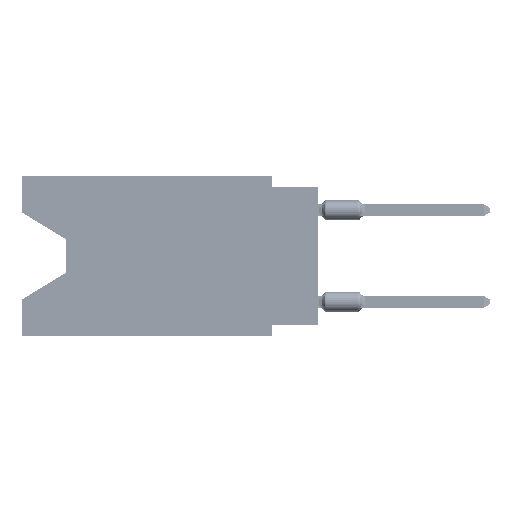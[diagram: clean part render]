
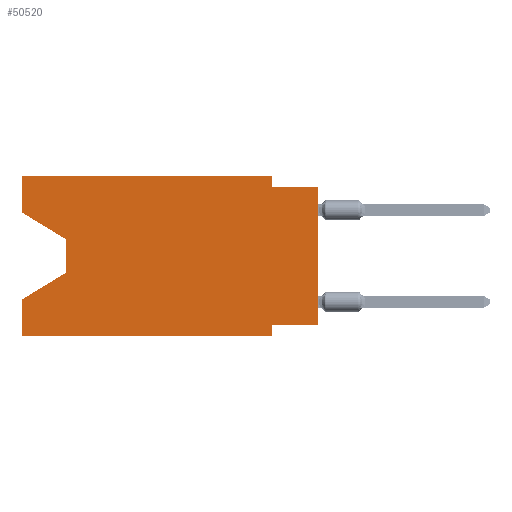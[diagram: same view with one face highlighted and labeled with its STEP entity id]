
A CAD part, left-side view. The second image highlights one B-rep face of the part: STEP entity #50520.
In plain terms, the highlighted planar face has unit normal (-1, 0, 0).
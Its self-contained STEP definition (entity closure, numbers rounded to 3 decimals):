
#161 = LINE ( 'NONE', #12127, #53376 ) ;
#1389 = VECTOR ( 'NONE', #43914, 1000. ) ;
#1641 = LINE ( 'NONE', #44809, #1389 ) ;
#2248 = EDGE_LOOP ( 'NONE', ( #59812, #13426, #54206, #58978, #23460, #26649, #7965, #26960, #28884, #45983, #70749, #5199 ) ) ;
#3345 = VECTOR ( 'NONE', #57295, 1000. ) ;
#5199 = ORIENTED_EDGE ( 'NONE', *, *, #15445, .F. ) ;
#7042 = DIRECTION ( 'NONE',  ( 0., 0., 1. ) ) ;
#7626 = DIRECTION ( 'NONE',  ( 0., 0.855, -0.519 ) ) ;
#7965 = ORIENTED_EDGE ( 'NONE', *, *, #70146, .F. ) ;
#9611 = VECTOR ( 'NONE', #7626, 1000. ) ;
#10541 = CARTESIAN_POINT ( 'NONE',  ( 0., 0., -0.635 ) ) ;
#10916 = DIRECTION ( 'NONE',  ( 0., 1., 0. ) ) ;
#10945 = DIRECTION ( 'NONE',  ( 0., -1., 0. ) ) ;
#11684 = VECTOR ( 'NONE', #10916, 1000. ) ;
#12127 = CARTESIAN_POINT ( 'NONE',  ( 0., 16.383, 0. ) ) ;
#12243 = VECTOR ( 'NONE', #10945, 1000. ) ;
#12475 = EDGE_CURVE ( 'NONE', #48709, #77872, #28798, .T. ) ;
#13426 = ORIENTED_EDGE ( 'NONE', *, *, #64429, .T. ) ;
#15445 = EDGE_CURVE ( 'NONE', #65819, #48709, #1641, .T. ) ;
#17161 = DIRECTION ( 'NONE',  ( 0., 0., -1. ) ) ;
#17624 = LINE ( 'NONE', #74138, #35516 ) ;
#19048 = LINE ( 'NONE', #75562, #59795 ) ;
#19210 = LINE ( 'NONE', #73902, #12243 ) ;
#19377 = CARTESIAN_POINT ( 'NONE',  ( 0., 2.54, -8.255 ) ) ;
#19609 = AXIS2_PLACEMENT_3D ( 'NONE', #20491, #35161, #41598 ) ;
#20093 = VECTOR ( 'NONE', #58358, 1000. ) ;
#20491 = CARTESIAN_POINT ( 'NONE',  ( 0., 16.383, 0. ) ) ;
#23460 = ORIENTED_EDGE ( 'NONE', *, *, #77957, .T. ) ;
#25932 = DIRECTION ( 'NONE',  ( 0., -0.855, -0.519 ) ) ;
#26649 = ORIENTED_EDGE ( 'NONE', *, *, #27356, .F. ) ;
#26960 = ORIENTED_EDGE ( 'NONE', *, *, #90694, .T. ) ;
#27356 = EDGE_CURVE ( 'NONE', #56264, #39975, #40721, .T. ) ;
#27609 = CARTESIAN_POINT ( 'NONE',  ( 0., 13.97, -3.505 ) ) ;
#28172 = CARTESIAN_POINT ( 'NONE',  ( 0., 16.383, -2.038 ) ) ;
#28798 = LINE ( 'NONE', #78430, #3345 ) ;
#28884 = ORIENTED_EDGE ( 'NONE', *, *, #64665, .F. ) ;
#30377 = VERTEX_POINT ( 'NONE', #51569 ) ;
#30771 = LINE ( 'NONE', #10541, #20093 ) ;
#31588 = CARTESIAN_POINT ( 'NONE',  ( 0., 16.383, -6.852 ) ) ;
#32415 = CARTESIAN_POINT ( 'NONE',  ( 0., 0., -0.635 ) ) ;
#35161 = DIRECTION ( 'NONE',  ( 1., 0., 0. ) ) ;
#35516 = VECTOR ( 'NONE', #17161, 1000. ) ;
#36182 = VERTEX_POINT ( 'NONE', #31588 ) ;
#36386 = LINE ( 'NONE', #86483, #37163 ) ;
#37163 = VECTOR ( 'NONE', #50186, 1000. ) ;
#39975 = VERTEX_POINT ( 'NONE', #74692 ) ;
#40721 = LINE ( 'NONE', #54986, #90633 ) ;
#41598 = DIRECTION ( 'NONE',  ( 0., 0., -1. ) ) ;
#43440 = CARTESIAN_POINT ( 'NONE',  ( 0., 13.97, -3.505 ) ) ;
#43914 = DIRECTION ( 'NONE',  ( 0., 0., 1. ) ) ;
#44809 = CARTESIAN_POINT ( 'NONE',  ( 0., 16.383, 0. ) ) ;
#45229 = VECTOR ( 'NONE', #55647, 1000. ) ;
#45983 = ORIENTED_EDGE ( 'NONE', *, *, #89313, .F. ) ;
#48709 = VERTEX_POINT ( 'NONE', #75451 ) ;
#49525 = CARTESIAN_POINT ( 'NONE',  ( 0., 16.383, -8.89 ) ) ;
#50186 = DIRECTION ( 'NONE',  ( 0., 0., 1. ) ) ;
#50520 = ADVANCED_FACE ( 'NONE', ( #90780 ), #83452, .F. ) ;
#51569 = CARTESIAN_POINT ( 'NONE',  ( 0., 0., -8.255 ) ) ;
#52077 = EDGE_CURVE ( 'NONE', #58497, #36182, #161, .T. ) ;
#52764 = CARTESIAN_POINT ( 'NONE',  ( 0., 2.54, 0. ) ) ;
#52921 = LINE ( 'NONE', #27609, #45229 ) ;
#53376 = VECTOR ( 'NONE', #7042, 1000. ) ;
#53477 = VERTEX_POINT ( 'NONE', #43440 ) ;
#53838 = CARTESIAN_POINT ( 'NONE',  ( 0., 2.54, -0.635 ) ) ;
#54206 = ORIENTED_EDGE ( 'NONE', *, *, #81748, .T. ) ;
#54986 = CARTESIAN_POINT ( 'NONE',  ( 0., 2.54, -8.89 ) ) ;
#55239 = VERTEX_POINT ( 'NONE', #65712 ) ;
#55647 = DIRECTION ( 'NONE',  ( 0., 0., -1. ) ) ;
#56264 = VERTEX_POINT ( 'NONE', #19377 ) ;
#57295 = DIRECTION ( 'NONE',  ( 0., -1., 0. ) ) ;
#58358 = DIRECTION ( 'NONE',  ( 0., -1., 0. ) ) ;
#58497 = VERTEX_POINT ( 'NONE', #49525 ) ;
#58978 = ORIENTED_EDGE ( 'NONE', *, *, #52077, .F. ) ;
#59189 = LINE ( 'NONE', #79872, #11684 ) ;
#59795 = VECTOR ( 'NONE', #25932, 1000. ) ;
#59812 = ORIENTED_EDGE ( 'NONE', *, *, #85480, .T. ) ;
#64429 = EDGE_CURVE ( 'NONE', #53477, #55239, #52921, .T. ) ;
#64665 = EDGE_CURVE ( 'NONE', #69333, #76208, #30771, .T. ) ;
#65712 = CARTESIAN_POINT ( 'NONE',  ( 0., 13.97, -5.385 ) ) ;
#65819 = VERTEX_POINT ( 'NONE', #28172 ) ;
#68768 = DIRECTION ( 'NONE',  ( 0., 0., -1. ) ) ;
#69333 = VERTEX_POINT ( 'NONE', #53838 ) ;
#70146 = EDGE_CURVE ( 'NONE', #30377, #56264, #59189, .T. ) ;
#70749 = ORIENTED_EDGE ( 'NONE', *, *, #12475, .F. ) ;
#73902 = CARTESIAN_POINT ( 'NONE',  ( 0., 16.383, -8.89 ) ) ;
#74138 = CARTESIAN_POINT ( 'NONE',  ( 0., 2.54, 0. ) ) ;
#74692 = CARTESIAN_POINT ( 'NONE',  ( 0., 2.54, -8.89 ) ) ;
#75451 = CARTESIAN_POINT ( 'NONE',  ( 0., 16.383, 0. ) ) ;
#75562 = CARTESIAN_POINT ( 'NONE',  ( 0., 16.383, -2.038 ) ) ;
#76208 = VERTEX_POINT ( 'NONE', #32415 ) ;
#77486 = LINE ( 'NONE', #85740, #9611 ) ;
#77872 = VERTEX_POINT ( 'NONE', #52764 ) ;
#77957 = EDGE_CURVE ( 'NONE', #58497, #39975, #19210, .T. ) ;
#78430 = CARTESIAN_POINT ( 'NONE',  ( 0., 16.383, 0. ) ) ;
#79872 = CARTESIAN_POINT ( 'NONE',  ( 0., 0., -8.255 ) ) ;
#81748 = EDGE_CURVE ( 'NONE', #55239, #36182, #77486, .T. ) ;
#83452 = PLANE ( 'NONE',  #19609 ) ;
#85480 = EDGE_CURVE ( 'NONE', #65819, #53477, #19048, .T. ) ;
#85740 = CARTESIAN_POINT ( 'NONE',  ( 0., 13.97, -5.385 ) ) ;
#86483 = CARTESIAN_POINT ( 'NONE',  ( 0., 0., 0. ) ) ;
#89313 = EDGE_CURVE ( 'NONE', #77872, #69333, #17624, .T. ) ;
#90633 = VECTOR ( 'NONE', #68768, 1000. ) ;
#90694 = EDGE_CURVE ( 'NONE', #30377, #76208, #36386, .T. ) ;
#90780 = FACE_OUTER_BOUND ( 'NONE', #2248, .T. ) ;
